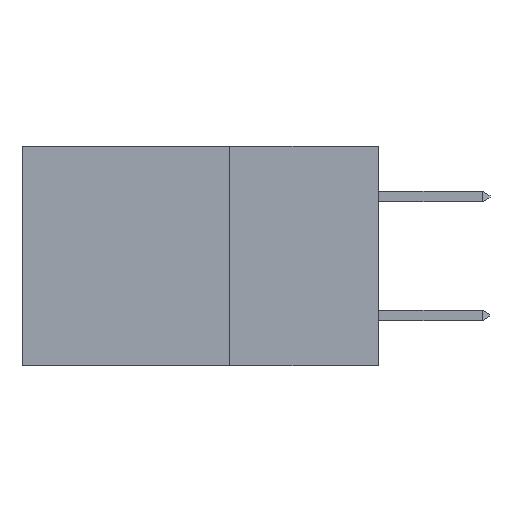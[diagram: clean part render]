
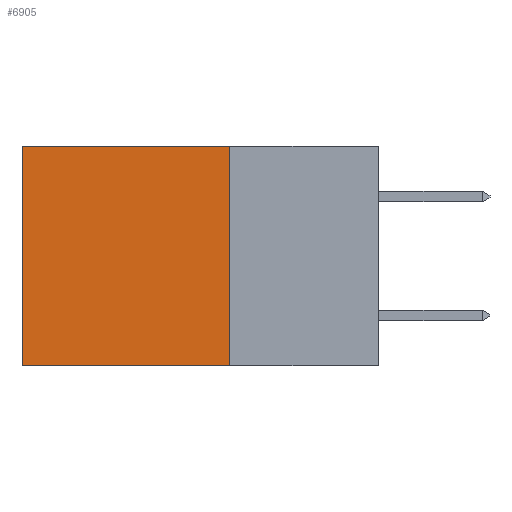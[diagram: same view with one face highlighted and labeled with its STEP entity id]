
A CAD part, left-side view. The second image highlights one B-rep face of the part: STEP entity #6905.
In plain terms, the highlighted planar face has unit normal (-1, 0, 0).
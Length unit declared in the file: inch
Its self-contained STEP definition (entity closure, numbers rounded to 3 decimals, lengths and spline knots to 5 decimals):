
#601 = VECTOR ( 'NONE', #12927, 39.37008 ) ;
#1137 = EDGE_CURVE ( 'NONE', #11151, #1372, #7324, .T. ) ;
#1372 = VERTEX_POINT ( 'NONE', #4630 ) ;
#1494 = DIRECTION ( 'NONE',  ( 0., 0., -1. ) ) ;
#1847 = CARTESIAN_POINT ( 'NONE',  ( 0.298, 0.6, 0. ) ) ;
#2238 = ORIENTED_EDGE ( 'NONE', *, *, #1137, .F. ) ;
#2763 = VECTOR ( 'NONE', #15587, 39.37008 ) ;
#3023 = EDGE_LOOP ( 'NONE', ( #13739, #12663, #2238, #17858 ) ) ;
#3113 = FACE_OUTER_BOUND ( 'NONE', #3023, .T. ) ;
#4630 = CARTESIAN_POINT ( 'NONE',  ( 0.298, 0.25, -0.37 ) ) ;
#4636 = EDGE_CURVE ( 'NONE', #1372, #8022, #5637, .T. ) ;
#4671 = VECTOR ( 'NONE', #13186, 39.37008 ) ;
#5637 = LINE ( 'NONE', #10024, #4671 ) ;
#6905 = ADVANCED_FACE ( 'NONE', ( #3113 ), #19765, .F. ) ;
#7042 = CARTESIAN_POINT ( 'NONE',  ( 0.298, 0.6, 0. ) ) ;
#7324 = LINE ( 'NONE', #14251, #2763 ) ;
#8022 = VERTEX_POINT ( 'NONE', #11667 ) ;
#8554 = EDGE_CURVE ( 'NONE', #11151, #17626, #12825, .T. ) ;
#9910 = LINE ( 'NONE', #7042, #13975 ) ;
#10024 = CARTESIAN_POINT ( 'NONE',  ( 0.298, 0.25, -0.37 ) ) ;
#10358 = AXIS2_PLACEMENT_3D ( 'NONE', #15235, #10660, #1494 ) ;
#10660 = DIRECTION ( 'NONE',  ( 1., 0., 0. ) ) ;
#11151 = VERTEX_POINT ( 'NONE', #15597 ) ;
#11667 = CARTESIAN_POINT ( 'NONE',  ( 0.298, 0.6, -0.37 ) ) ;
#12663 = ORIENTED_EDGE ( 'NONE', *, *, #4636, .F. ) ;
#12825 = LINE ( 'NONE', #17458, #601 ) ;
#12927 = DIRECTION ( 'NONE',  ( 0., 1., 0. ) ) ;
#13186 = DIRECTION ( 'NONE',  ( 0., 1., 0. ) ) ;
#13739 = ORIENTED_EDGE ( 'NONE', *, *, #15860, .T. ) ;
#13975 = VECTOR ( 'NONE', #17685, 39.37008 ) ;
#14251 = CARTESIAN_POINT ( 'NONE',  ( 0.298, 0.25, 0. ) ) ;
#15235 = CARTESIAN_POINT ( 'NONE',  ( 0.298, 0.25, 0. ) ) ;
#15587 = DIRECTION ( 'NONE',  ( 0., 0., -1. ) ) ;
#15597 = CARTESIAN_POINT ( 'NONE',  ( 0.298, 0.25, 0. ) ) ;
#15860 = EDGE_CURVE ( 'NONE', #17626, #8022, #9910, .T. ) ;
#17458 = CARTESIAN_POINT ( 'NONE',  ( 0.298, 0.25, 0. ) ) ;
#17626 = VERTEX_POINT ( 'NONE', #1847 ) ;
#17685 = DIRECTION ( 'NONE',  ( 0., 0., -1. ) ) ;
#17858 = ORIENTED_EDGE ( 'NONE', *, *, #8554, .T. ) ;
#19765 = PLANE ( 'NONE',  #10358 ) ;
